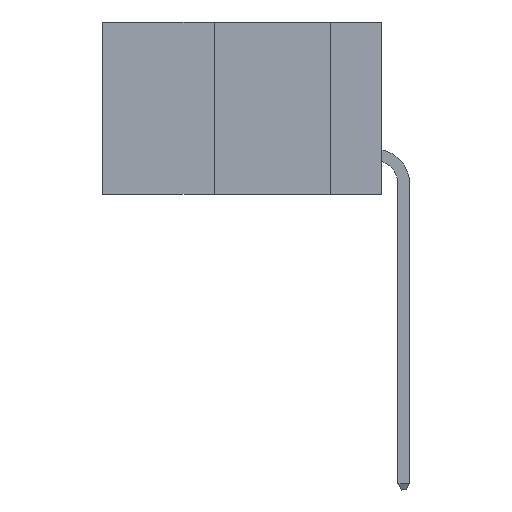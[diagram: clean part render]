
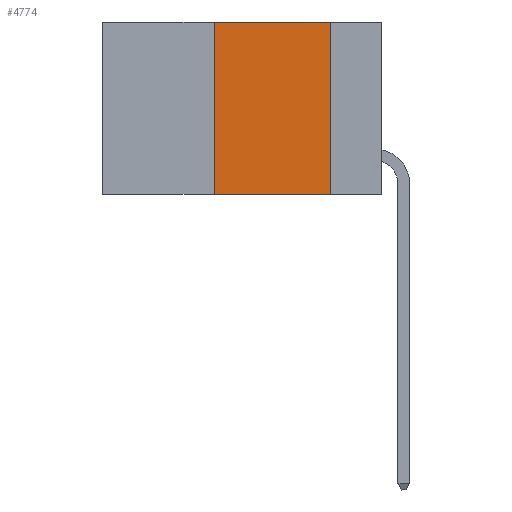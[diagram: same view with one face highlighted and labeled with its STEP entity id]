
A CAD part, left-side view. The second image highlights one B-rep face of the part: STEP entity #4774.
In plain terms, the highlighted planar face has unit normal (-1, 0, 0).
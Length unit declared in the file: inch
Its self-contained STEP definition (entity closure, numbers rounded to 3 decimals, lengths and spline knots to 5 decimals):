
#93 = CARTESIAN_POINT ( 'NONE',  ( 0., 0.36, 0. ) ) ;
#1044 = VECTOR ( 'NONE', #8695, 39.37008 ) ;
#1388 = EDGE_CURVE ( 'NONE', #5878, #4073, #3105, .T. ) ;
#2212 = CARTESIAN_POINT ( 'NONE',  ( 0., 0.6, -0.37 ) ) ;
#2349 = DIRECTION ( 'NONE',  ( 0., -1., 0. ) ) ;
#2525 = VERTEX_POINT ( 'NONE', #93 ) ;
#3105 = LINE ( 'NONE', #4530, #1044 ) ;
#3205 = CARTESIAN_POINT ( 'NONE',  ( 0., 0.11, -0.37 ) ) ;
#3791 = CARTESIAN_POINT ( 'NONE',  ( 0., 0.6, 0. ) ) ;
#3851 = VECTOR ( 'NONE', #8679, 39.37008 ) ;
#4063 = ORIENTED_EDGE ( 'NONE', *, *, #6196, .F. ) ;
#4073 = VERTEX_POINT ( 'NONE', #3205 ) ;
#4136 = FACE_OUTER_BOUND ( 'NONE', #5713, .T. ) ;
#4186 = EDGE_CURVE ( 'NONE', #4404, #4073, #8470, .T. ) ;
#4209 = CARTESIAN_POINT ( 'NONE',  ( 0., 0.36, -0.37 ) ) ;
#4348 = ORIENTED_EDGE ( 'NONE', *, *, #4186, .T. ) ;
#4404 = VERTEX_POINT ( 'NONE', #4209 ) ;
#4530 = CARTESIAN_POINT ( 'NONE',  ( 0., 0.11, 0. ) ) ;
#4774 = ADVANCED_FACE ( 'NONE', ( #4136 ), #7789, .F. ) ;
#5181 = EDGE_CURVE ( 'NONE', #4404, #2525, #9550, .T. ) ;
#5713 = EDGE_LOOP ( 'NONE', ( #5993, #4063, #6186, #4348 ) ) ;
#5878 = VERTEX_POINT ( 'NONE', #6071 ) ;
#5993 = ORIENTED_EDGE ( 'NONE', *, *, #1388, .F. ) ;
#6071 = CARTESIAN_POINT ( 'NONE',  ( 0., 0.11, 0. ) ) ;
#6186 = ORIENTED_EDGE ( 'NONE', *, *, #5181, .F. ) ;
#6196 = EDGE_CURVE ( 'NONE', #2525, #5878, #8523, .T. ) ;
#6206 = DIRECTION ( 'NONE',  ( 0., -1., 0. ) ) ;
#6313 = VECTOR ( 'NONE', #6206, 39.37008 ) ;
#6684 = VECTOR ( 'NONE', #2349, 39.37008 ) ;
#7204 = AXIS2_PLACEMENT_3D ( 'NONE', #7808, #8905, #7780 ) ;
#7780 = DIRECTION ( 'NONE',  ( 0., 0., -1. ) ) ;
#7789 = PLANE ( 'NONE',  #7204 ) ;
#7808 = CARTESIAN_POINT ( 'NONE',  ( 0., 0.6, 0. ) ) ;
#8462 = CARTESIAN_POINT ( 'NONE',  ( 0., 0.36, 0. ) ) ;
#8470 = LINE ( 'NONE', #2212, #6684 ) ;
#8523 = LINE ( 'NONE', #3791, #6313 ) ;
#8679 = DIRECTION ( 'NONE',  ( 0., 0., 1. ) ) ;
#8695 = DIRECTION ( 'NONE',  ( 0., 0., -1. ) ) ;
#8905 = DIRECTION ( 'NONE',  ( 1., 0., 0. ) ) ;
#9550 = LINE ( 'NONE', #8462, #3851 ) ;
